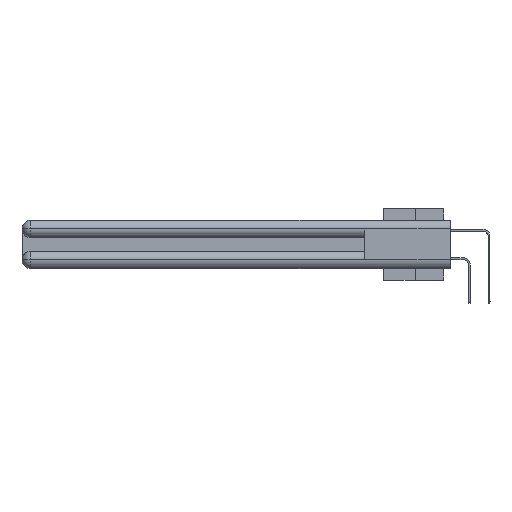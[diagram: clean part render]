
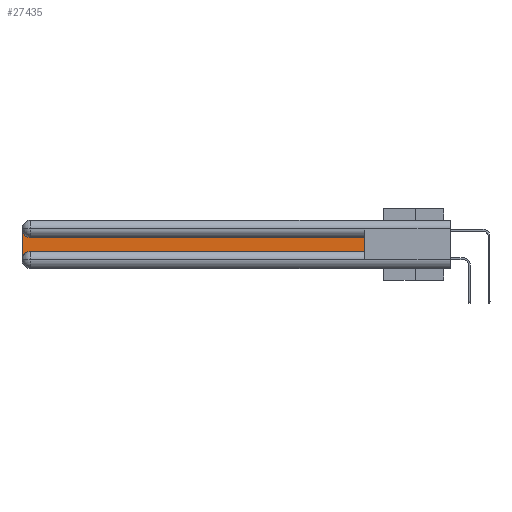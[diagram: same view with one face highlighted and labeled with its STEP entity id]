
A CAD part, left-side view. The second image highlights one B-rep face of the part: STEP entity #27435.
In plain terms, the highlighted planar face has unit normal (-1, 0, 0).
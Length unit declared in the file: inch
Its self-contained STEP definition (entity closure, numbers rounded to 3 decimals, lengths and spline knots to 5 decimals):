
#159 = ORIENTED_EDGE ( 'NONE', *, *, #13847, .T. ) ;
#1236 = AXIS2_PLACEMENT_3D ( 'NONE', #21221, #31833, #4427 ) ;
#1841 = CARTESIAN_POINT ( 'NONE',  ( 0.075, 2.94, -0.0625 ) ) ;
#2029 = CARTESIAN_POINT ( 'NONE',  ( 0.075, 0.6, -0.1225 ) ) ;
#2979 = DIRECTION ( 'NONE',  ( 0., 0., 1. ) ) ;
#3383 = LINE ( 'NONE', #9993, #9509 ) ;
#3785 = VERTEX_POINT ( 'NONE', #29077 ) ;
#4419 = ORIENTED_EDGE ( 'NONE', *, *, #31641, .T. ) ;
#4427 = DIRECTION ( 'NONE',  ( 0., 0., -1. ) ) ;
#5389 = EDGE_LOOP ( 'NONE', ( #12198, #33089, #4419, #29153, #159, #17601 ) ) ;
#6059 = CARTESIAN_POINT ( 'NONE',  ( 0.075, 0.6, -0.1225 ) ) ;
#8293 = VERTEX_POINT ( 'NONE', #27476 ) ;
#9324 = CARTESIAN_POINT ( 'NONE',  ( 0.075, 2.94, -0.2775 ) ) ;
#9509 = VECTOR ( 'NONE', #15569, 39.37008 ) ;
#9993 = CARTESIAN_POINT ( 'NONE',  ( 0.075, 3., -0.2175 ) ) ;
#10148 = CIRCLE ( 'NONE', #26119, 0.06 ) ;
#10180 = CARTESIAN_POINT ( 'NONE',  ( 0.075, 2.94, -0.2175 ) ) ;
#10730 = LINE ( 'NONE', #6059, #20719 ) ;
#12058 = VECTOR ( 'NONE', #22219, 39.37008 ) ;
#12198 = ORIENTED_EDGE ( 'NONE', *, *, #34781, .T. ) ;
#13847 = EDGE_CURVE ( 'NONE', #33343, #23654, #21626, .T. ) ;
#14632 = FACE_OUTER_BOUND ( 'NONE', #5389, .T. ) ;
#15252 = LINE ( 'NONE', #32809, #25698 ) ;
#15265 = PLANE ( 'NONE',  #1236 ) ;
#15569 = DIRECTION ( 'NONE',  ( 0., 0., -1. ) ) ;
#16256 = CARTESIAN_POINT ( 'NONE',  ( 0.075, 0.6, -0.2175 ) ) ;
#16627 = DIRECTION ( 'NONE',  ( 0., 1., 0. ) ) ;
#16740 = CIRCLE ( 'NONE', #19590, 0.06 ) ;
#17601 = ORIENTED_EDGE ( 'NONE', *, *, #30401, .T. ) ;
#17703 = DIRECTION ( 'NONE',  ( 0., 0., -1. ) ) ;
#18160 = VERTEX_POINT ( 'NONE', #24874 ) ;
#19576 = EDGE_CURVE ( 'NONE', #3785, #33343, #10148, .T. ) ;
#19590 = AXIS2_PLACEMENT_3D ( 'NONE', #1841, #35556, #29603 ) ;
#20719 = VECTOR ( 'NONE', #16627, 39.37008 ) ;
#21221 = CARTESIAN_POINT ( 'NONE',  ( 0.075, 3., -0.1225 ) ) ;
#21626 = LINE ( 'NONE', #16256, #12058 ) ;
#22219 = DIRECTION ( 'NONE',  ( 0., -1., 0. ) ) ;
#23654 = VERTEX_POINT ( 'NONE', #33984 ) ;
#23951 = EDGE_CURVE ( 'NONE', #18160, #8293, #16740, .T. ) ;
#24874 = CARTESIAN_POINT ( 'NONE',  ( 0.075, 2.94, -0.1225 ) ) ;
#25698 = VECTOR ( 'NONE', #2979, 39.37008 ) ;
#25709 = VERTEX_POINT ( 'NONE', #2029 ) ;
#26119 = AXIS2_PLACEMENT_3D ( 'NONE', #9324, #28811, #17703 ) ;
#27435 = ADVANCED_FACE ( 'NONE', ( #14632 ), #15265, .F. ) ;
#27476 = CARTESIAN_POINT ( 'NONE',  ( 0.075, 3., -0.0625 ) ) ;
#28811 = DIRECTION ( 'NONE',  ( 1., 0., 0. ) ) ;
#29077 = CARTESIAN_POINT ( 'NONE',  ( 0.075, 3., -0.2775 ) ) ;
#29153 = ORIENTED_EDGE ( 'NONE', *, *, #19576, .T. ) ;
#29603 = DIRECTION ( 'NONE',  ( 0., 0., -1. ) ) ;
#30401 = EDGE_CURVE ( 'NONE', #23654, #25709, #15252, .T. ) ;
#31641 = EDGE_CURVE ( 'NONE', #8293, #3785, #3383, .T. ) ;
#31833 = DIRECTION ( 'NONE',  ( 1., 0., 0. ) ) ;
#32809 = CARTESIAN_POINT ( 'NONE',  ( 0.075, 0.6, -0.2175 ) ) ;
#33089 = ORIENTED_EDGE ( 'NONE', *, *, #23951, .T. ) ;
#33343 = VERTEX_POINT ( 'NONE', #10180 ) ;
#33984 = CARTESIAN_POINT ( 'NONE',  ( 0.075, 0.6, -0.2175 ) ) ;
#34781 = EDGE_CURVE ( 'NONE', #25709, #18160, #10730, .T. ) ;
#35556 = DIRECTION ( 'NONE',  ( 1., 0., 0. ) ) ;
